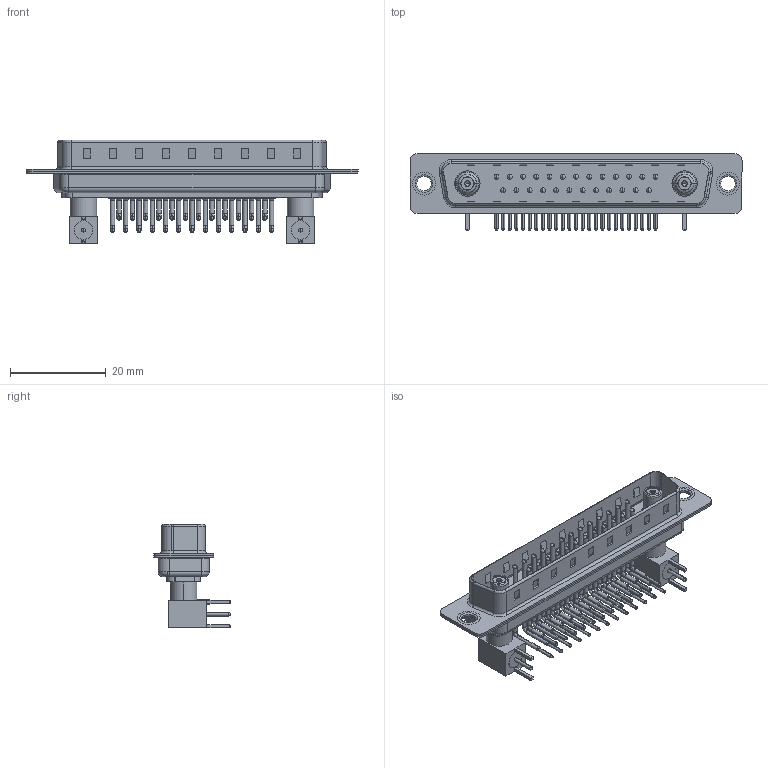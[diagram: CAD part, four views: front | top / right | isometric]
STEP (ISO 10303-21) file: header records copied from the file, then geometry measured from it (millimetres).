
FILE_DESCRIPTION (( 'STEP AP203' ), '1' );
FILE_NAME ('629-27W2640-5T1.STEP', '2022-05-16T19:37:17', ( '' ), ( '' ), 'SwSTEP 2.0', 'SolidWorks 2020', '' );
FILE_SCHEMA (( 'CONFIG_CONTROL_DESIGN' ));
Length unit declared in the file: millimetre
Products named in the file (16): Co-Ax Jack_RA PC Tail; Locking Collar; Co-Ax Jack Assy_RA; 629-27W2640-5T1; 629Combo Shell Rear_37 Contacts; 629Combo Thru Hole Rivet; 629Combo Contact Row 1; Insulator Socket 2; 629Combo Housing_27W2; 629Combo Shell Front_37 Contacts; Insulator RA Pin; 629Combo Contact Row 2; RA Back Shell; Socket_RA; Insulator Socket
Assembly tree (46 placements, depth 3):
  629-27W2640-5T1
    629Combo Housing_27W2
    629Combo Shell Rear_37 Contacts
    629Combo Shell Front_37 Contacts
    629Combo Thru Hole Rivet  x2
    Co-Ax Jack Assy_RA
      Co-Ax Jack_RA PC Tail
      Insulator Socket
      Insulator Socket 2
      Locking Collar
      Socket_RA
      RA Back Shell
      Insulator RA Pin
    Co-Ax Jack Assy_RA
      Co-Ax Jack_RA PC Tail
      Insulator Socket
      Insulator Socket 2
      Locking Collar
      Socket_RA
      RA Back Shell
      Insulator RA Pin
    629Combo Contact Row 1  x13
    629Combo Contact Row 2  x12
Bounding box: 69.4 x 16 x 21.71 mm (x, y, z)
Volume: 4457.5 mm3; surface area: 11644.9 mm2
Topology: 44 solids, 44 shells, 3440 faces, 9441 edges, 6112 vertices
Faces by surface type: plane 1917, cylinder 1159, bspline 152, cone 138, torus 70, sphere 4
Entity records: 30953 total; most frequent: CARTESIAN_POINT 5212, DIRECTION 5125, ORIENTED_EDGE 4616, EDGE_CURVE 2308, AXIS2_PLACEMENT_3D 1885, VERTEX_POINT 1487, LINE 1355, VECTOR 1355
